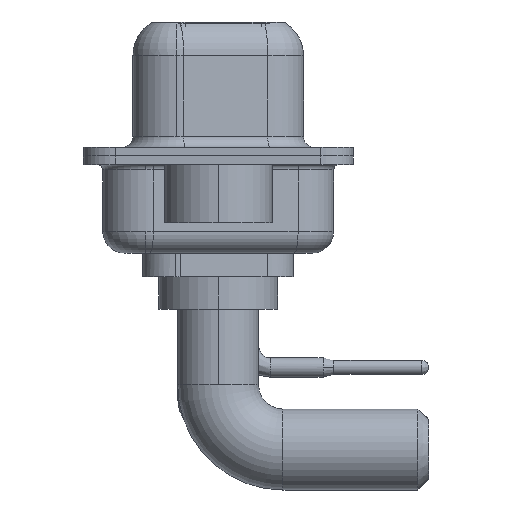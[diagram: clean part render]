
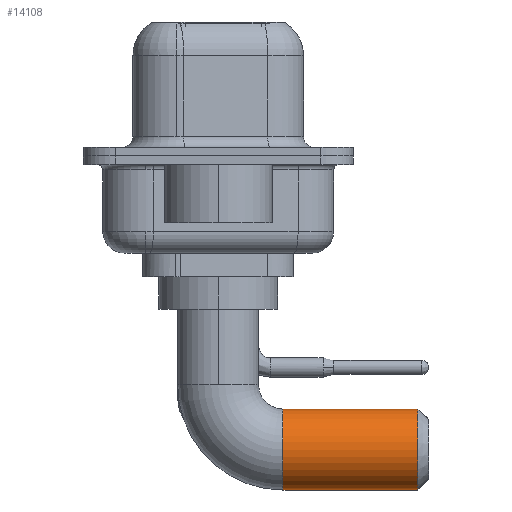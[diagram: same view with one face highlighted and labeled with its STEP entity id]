
A CAD part, left-side view. The second image highlights one B-rep face of the part: STEP entity #14108.
In plain terms, the highlighted cylindrical face has radius 1.875 mm (diameter 3.75 mm), a partial arc.
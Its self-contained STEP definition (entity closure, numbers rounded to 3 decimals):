
#663 = AXIS2_PLACEMENT_3D ( 'NONE', #8919, #897, #2387 ) ;
#897 = DIRECTION ( 'NONE',  ( 0., -1., 0. ) ) ;
#2382 = CIRCLE ( 'NONE', #19912, 1.875 ) ;
#2387 = DIRECTION ( 'NONE',  ( 0., 0., -1. ) ) ;
#2479 = DIRECTION ( 'NONE',  ( 0., -1., 0. ) ) ;
#2493 = CYLINDRICAL_SURFACE ( 'NONE', #663, 1.875 ) ;
#2628 = CARTESIAN_POINT ( 'NONE',  ( 0., -3., -4.625 ) ) ;
#3657 = CARTESIAN_POINT ( 'NONE',  ( 0., -9.25, -8.375 ) ) ;
#4058 = CARTESIAN_POINT ( 'NONE',  ( 0., -3., -6.5 ) ) ;
#5392 = VERTEX_POINT ( 'NONE', #12611 ) ;
#5812 = DIRECTION ( 'NONE',  ( 0., -1., 0. ) ) ;
#6152 = EDGE_LOOP ( 'NONE', ( #14955, #7500, #18833, #10597 ) ) ;
#6819 = VERTEX_POINT ( 'NONE', #8486 ) ;
#7500 = ORIENTED_EDGE ( 'NONE', *, *, #15686, .T. ) ;
#7560 = VECTOR ( 'NONE', #5812, 1000. ) ;
#7862 = DIRECTION ( 'NONE',  ( 0., -1., 0. ) ) ;
#8064 = DIRECTION ( 'NONE',  ( 0., 1., 0. ) ) ;
#8486 = CARTESIAN_POINT ( 'NONE',  ( 0., -9.25, -4.625 ) ) ;
#8919 = CARTESIAN_POINT ( 'NONE',  ( 0., -3., -6.5 ) ) ;
#10597 = ORIENTED_EDGE ( 'NONE', *, *, #15868, .T. ) ;
#11159 = CIRCLE ( 'NONE', #20256, 1.875 ) ;
#12200 = FACE_OUTER_BOUND ( 'NONE', #6152, .T. ) ;
#12611 = CARTESIAN_POINT ( 'NONE',  ( 0., -3., -8.375 ) ) ;
#13614 = VERTEX_POINT ( 'NONE', #2628 ) ;
#14092 = LINE ( 'NONE', #15987, #17188 ) ;
#14108 = ADVANCED_FACE ( 'NONE', ( #12200 ), #2493, .T. ) ;
#14261 = EDGE_CURVE ( 'NONE', #13614, #6819, #14092, .T. ) ;
#14610 = CARTESIAN_POINT ( 'NONE',  ( 0., -9.25, -6.5 ) ) ;
#14955 = ORIENTED_EDGE ( 'NONE', *, *, #14261, .F. ) ;
#15346 = DIRECTION ( 'NONE',  ( -1., 0., 0. ) ) ;
#15522 = CARTESIAN_POINT ( 'NONE',  ( 0., -3., -8.375 ) ) ;
#15686 = EDGE_CURVE ( 'NONE', #13614, #5392, #2382, .T. ) ;
#15868 = EDGE_CURVE ( 'NONE', #18781, #6819, #11159, .T. ) ;
#15987 = CARTESIAN_POINT ( 'NONE',  ( 0., -3., -4.625 ) ) ;
#16297 = DIRECTION ( 'NONE',  ( 0., 0., -1. ) ) ;
#17188 = VECTOR ( 'NONE', #7862, 1000. ) ;
#18781 = VERTEX_POINT ( 'NONE', #3657 ) ;
#18833 = ORIENTED_EDGE ( 'NONE', *, *, #19226, .T. ) ;
#19226 = EDGE_CURVE ( 'NONE', #5392, #18781, #20278, .T. ) ;
#19912 = AXIS2_PLACEMENT_3D ( 'NONE', #4058, #2479, #15346 ) ;
#20256 = AXIS2_PLACEMENT_3D ( 'NONE', #14610, #8064, #16297 ) ;
#20278 = LINE ( 'NONE', #15522, #7560 ) ;
